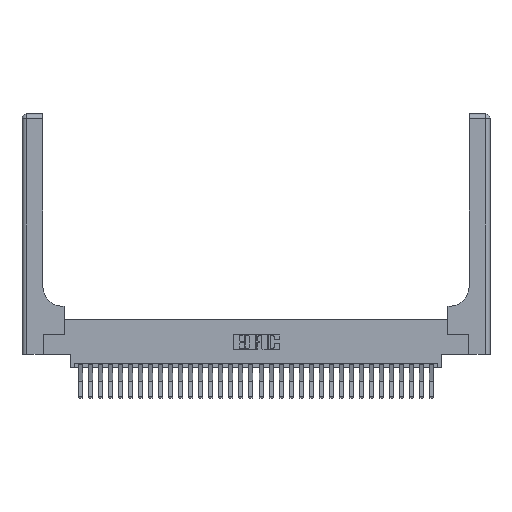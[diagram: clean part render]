
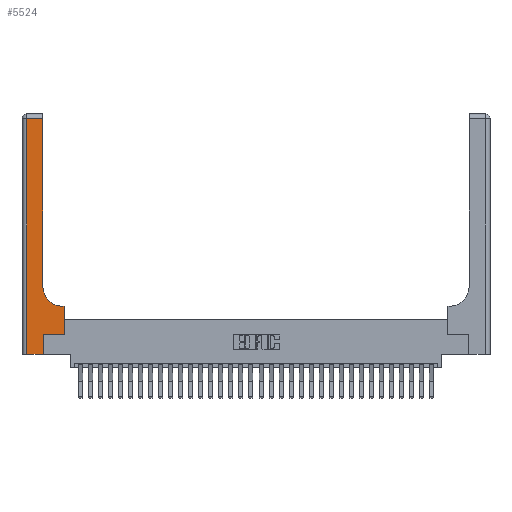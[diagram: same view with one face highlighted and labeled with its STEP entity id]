
A CAD part, top view. The second image highlights one B-rep face of the part: STEP entity #5524.
In plain terms, the highlighted planar face has unit normal (0, 0, 1).
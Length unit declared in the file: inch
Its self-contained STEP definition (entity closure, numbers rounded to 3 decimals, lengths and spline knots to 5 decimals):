
#302 = CARTESIAN_POINT ( 'NONE',  ( 0.06, 2.94, 0.37 ) ) ;
#506 = ORIENTED_EDGE ( 'NONE', *, *, #862, .T. ) ;
#862 = EDGE_CURVE ( 'NONE', #27035, #25067, #4532, .T. ) ;
#1589 = DIRECTION ( 'NONE',  ( 1., 0., 0. ) ) ;
#1632 = ORIENTED_EDGE ( 'NONE', *, *, #26256, .T. ) ;
#1955 = VECTOR ( 'NONE', #12861, 39.37008 ) ;
#2173 = DIRECTION ( 'NONE',  ( -1., 0., 0. ) ) ;
#2449 = LINE ( 'NONE', #20364, #13904 ) ;
#3206 = AXIS2_PLACEMENT_3D ( 'NONE', #8881, #15861, #2173 ) ;
#3705 = ORIENTED_EDGE ( 'NONE', *, *, #28690, .T. ) ;
#3755 = FACE_OUTER_BOUND ( 'NONE', #24002, .T. ) ;
#3912 = CARTESIAN_POINT ( 'NONE',  ( 0., 0., 0.37 ) ) ;
#4034 = VECTOR ( 'NONE', #1589, 39.37008 ) ;
#4532 = CIRCLE ( 'NONE', #7531, 0.25 ) ;
#4944 = CARTESIAN_POINT ( 'NONE',  ( 0.265, 0., 0.37 ) ) ;
#5465 = VECTOR ( 'NONE', #11991, 39.37008 ) ;
#5524 = ADVANCED_FACE ( 'NONE', ( #3755 ), #25054, .F. ) ;
#5710 = CARTESIAN_POINT ( 'NONE',  ( 0.06, 0., 0.37 ) ) ;
#6252 = EDGE_CURVE ( 'NONE', #26895, #25841, #9117, .T. ) ;
#7236 = EDGE_CURVE ( 'NONE', #12929, #27035, #20550, .T. ) ;
#7531 = AXIS2_PLACEMENT_3D ( 'NONE', #25602, #11817, #27886 ) ;
#8400 = VECTOR ( 'NONE', #23283, 39.37008 ) ;
#8881 = CARTESIAN_POINT ( 'NONE',  ( 0., 3., 0.37 ) ) ;
#8938 = DIRECTION ( 'NONE',  ( 0., 1., 0. ) ) ;
#9117 = LINE ( 'NONE', #4944, #8400 ) ;
#9120 = VERTEX_POINT ( 'NONE', #5710 ) ;
#9245 = DIRECTION ( 'NONE',  ( -1., 0., 0. ) ) ;
#9516 = LINE ( 'NONE', #13917, #27157 ) ;
#10366 = ORIENTED_EDGE ( 'NONE', *, *, #11749, .T. ) ;
#11301 = CARTESIAN_POINT ( 'NONE',  ( 0.26, 0.6, 0.37 ) ) ;
#11712 = DIRECTION ( 'NONE',  ( 1., 0., 0. ) ) ;
#11749 = EDGE_CURVE ( 'NONE', #18912, #23234, #12830, .T. ) ;
#11817 = DIRECTION ( 'NONE',  ( 0., 0., -1. ) ) ;
#11991 = DIRECTION ( 'NONE',  ( 0., 1., 0. ) ) ;
#12830 = LINE ( 'NONE', #20688, #18907 ) ;
#12861 = DIRECTION ( 'NONE',  ( 0., -1., 0. ) ) ;
#12929 = VERTEX_POINT ( 'NONE', #27485 ) ;
#13170 = DIRECTION ( 'NONE',  ( -1., 0., 0. ) ) ;
#13647 = CARTESIAN_POINT ( 'NONE',  ( 0.26, 0.85, 0.37 ) ) ;
#13725 = VECTOR ( 'NONE', #13170, 39.37008 ) ;
#13897 = EDGE_CURVE ( 'NONE', #25841, #15214, #9516, .T. ) ;
#13904 = VECTOR ( 'NONE', #8938, 39.37008 ) ;
#13917 = CARTESIAN_POINT ( 'NONE',  ( 0.265, 0.25, 0.37 ) ) ;
#14128 = LINE ( 'NONE', #22186, #1955 ) ;
#14536 = CARTESIAN_POINT ( 'NONE',  ( 0.528, 0.25, 0.37 ) ) ;
#15214 = VERTEX_POINT ( 'NONE', #14536 ) ;
#15563 = ORIENTED_EDGE ( 'NONE', *, *, #13897, .T. ) ;
#15861 = DIRECTION ( 'NONE',  ( 0., 0., -1. ) ) ;
#16406 = CARTESIAN_POINT ( 'NONE',  ( 0.26, 2.94, 0.37 ) ) ;
#17022 = ORIENTED_EDGE ( 'NONE', *, *, #24881, .T. ) ;
#17643 = LINE ( 'NONE', #28062, #5465 ) ;
#17760 = EDGE_CURVE ( 'NONE', #25067, #18912, #17643, .T. ) ;
#18267 = ORIENTED_EDGE ( 'NONE', *, *, #6252, .T. ) ;
#18907 = VECTOR ( 'NONE', #9245, 39.37008 ) ;
#18912 = VERTEX_POINT ( 'NONE', #16406 ) ;
#19674 = CARTESIAN_POINT ( 'NONE',  ( 0.265, 0., 0.37 ) ) ;
#20364 = CARTESIAN_POINT ( 'NONE',  ( 0.528, 0.25, 0.37 ) ) ;
#20550 = LINE ( 'NONE', #11301, #13725 ) ;
#20688 = CARTESIAN_POINT ( 'NONE',  ( 0., 2.94, 0.37 ) ) ;
#20827 = ORIENTED_EDGE ( 'NONE', *, *, #17760, .T. ) ;
#22186 = CARTESIAN_POINT ( 'NONE',  ( 0.06, 3., 0.37 ) ) ;
#22503 = CARTESIAN_POINT ( 'NONE',  ( 0.51, 0.6, 0.37 ) ) ;
#23234 = VERTEX_POINT ( 'NONE', #302 ) ;
#23283 = DIRECTION ( 'NONE',  ( 0., 1., 0. ) ) ;
#24002 = EDGE_LOOP ( 'NONE', ( #20827, #10366, #17022, #1632, #18267, #15563, #3705, #24904, #506 ) ) ;
#24881 = EDGE_CURVE ( 'NONE', #23234, #9120, #14128, .T. ) ;
#24904 = ORIENTED_EDGE ( 'NONE', *, *, #7236, .T. ) ;
#25054 = PLANE ( 'NONE',  #3206 ) ;
#25067 = VERTEX_POINT ( 'NONE', #13647 ) ;
#25410 = CARTESIAN_POINT ( 'NONE',  ( 0.265, 0.25, 0.37 ) ) ;
#25602 = CARTESIAN_POINT ( 'NONE',  ( 0.51, 0.85, 0.37 ) ) ;
#25841 = VERTEX_POINT ( 'NONE', #25410 ) ;
#26256 = EDGE_CURVE ( 'NONE', #9120, #26895, #28426, .T. ) ;
#26895 = VERTEX_POINT ( 'NONE', #19674 ) ;
#27035 = VERTEX_POINT ( 'NONE', #22503 ) ;
#27157 = VECTOR ( 'NONE', #11712, 39.37008 ) ;
#27485 = CARTESIAN_POINT ( 'NONE',  ( 0.528, 0.6, 0.37 ) ) ;
#27886 = DIRECTION ( 'NONE',  ( 1., 0., 0. ) ) ;
#28062 = CARTESIAN_POINT ( 'NONE',  ( 0.26, 3., 0.37 ) ) ;
#28426 = LINE ( 'NONE', #3912, #4034 ) ;
#28690 = EDGE_CURVE ( 'NONE', #15214, #12929, #2449, .T. ) ;
